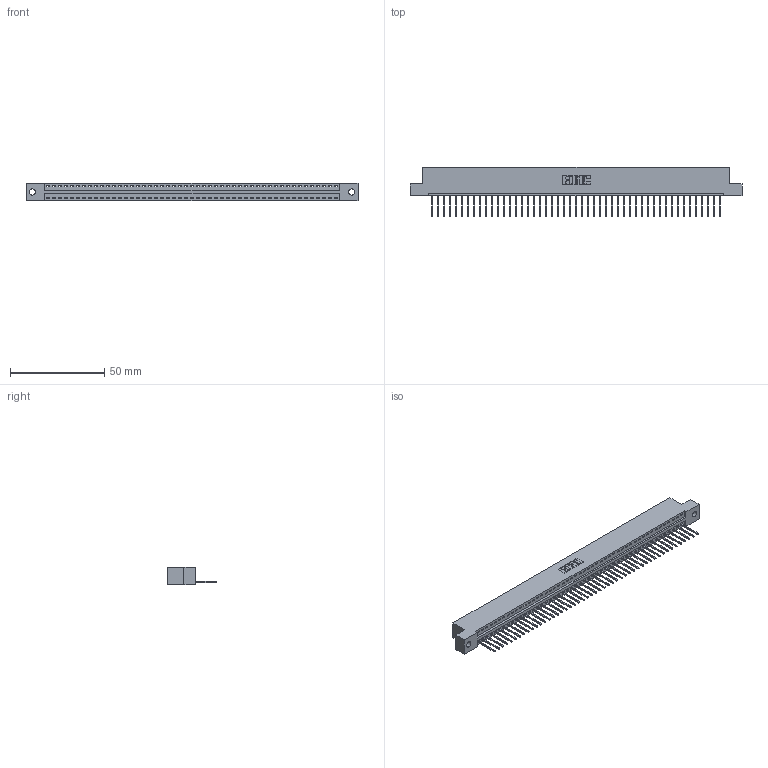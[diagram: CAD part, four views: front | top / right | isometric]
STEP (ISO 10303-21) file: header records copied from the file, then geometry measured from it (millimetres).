
FILE_DESCRIPTION (( 'STEP AP203' ), '1' );
FILE_NAME ('396-049-522-102.STEP', '2018-09-08T01:50:48', ( '' ), ( '' ), 'SwSTEP 2.0', 'SolidWorks 2016', '' );
FILE_SCHEMA (( 'CONFIG_CONTROL_DESIGN' ));
Length unit declared in the file: inch
Products named in the file (3): 345-292-001_345-293-122; 396-049-522-102; 346 Part_Flush Mounting Lugs - 0.128 Dia
Assembly tree (50 placements, depth 2):
  396-049-522-102
    346 Part_Flush Mounting Lugs - 0.128 Dia
    345-292-001_345-293-122  x49
Bounding box: 176.15 x 26.42 x 9.4 mm (x, y, z)
Volume: 16879 mm3; surface area: 21081.3 mm2
Topology: 50 solids, 50 shells, 2964 faces, 8953 edges, 5902 vertices
Faces by surface type: plane 2036, cylinder 928
Entity records: 29489 total; most frequent: CARTESIAN_POINT 5059, ORIENTED_EDGE 5042, DIRECTION 4455, EDGE_CURVE 2521, VECTOR 2193, LINE 2193, VERTEX_POINT 1678, AXIS2_PLACEMENT_3D 1131
